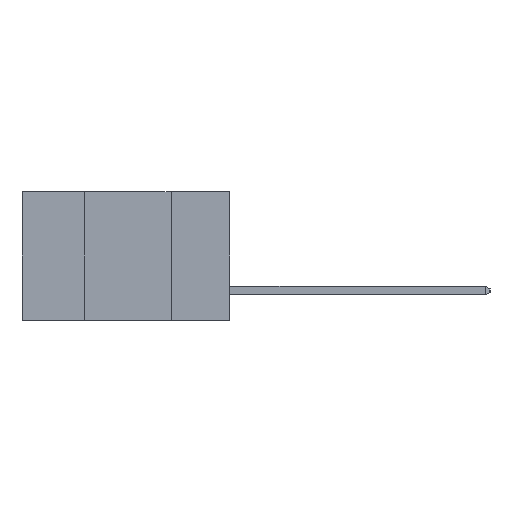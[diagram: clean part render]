
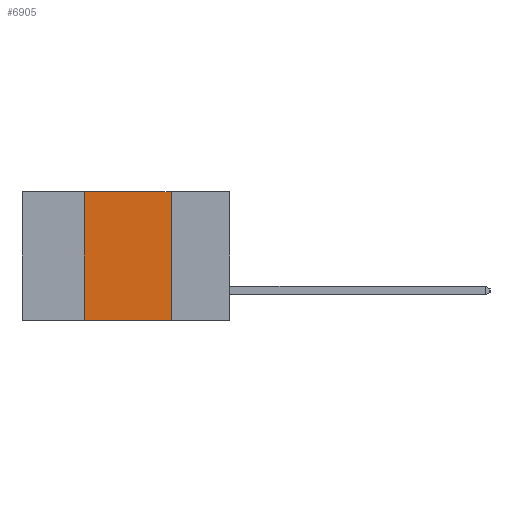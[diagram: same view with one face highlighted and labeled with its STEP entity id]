
A CAD part, left-side view. The second image highlights one B-rep face of the part: STEP entity #6905.
In plain terms, the highlighted planar face has unit normal (-1, 0, 0).
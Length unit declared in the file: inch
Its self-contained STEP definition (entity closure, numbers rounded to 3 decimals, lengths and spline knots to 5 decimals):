
#9 = DIRECTION ( 'NONE',  ( 0., 0., 1. ) ) ;
#81 = DIRECTION ( 'NONE',  ( 0., -1., 0. ) ) ;
#99 = VERTEX_POINT ( 'NONE', #8966 ) ;
#309 = VERTEX_POINT ( 'NONE', #1239 ) ;
#330 = VECTOR ( 'NONE', #81, 39.37008 ) ;
#433 = DIRECTION ( 'NONE',  ( 1., 0., 0. ) ) ;
#480 = DIRECTION ( 'NONE',  ( 0., 0., -1. ) ) ;
#745 = PLANE ( 'NONE',  #10791 ) ;
#835 = EDGE_CURVE ( 'NONE', #309, #99, #3803, .T. ) ;
#1147 = ORIENTED_EDGE ( 'NONE', *, *, #835, .F. ) ;
#1239 = CARTESIAN_POINT ( 'NONE',  ( 0., 0.42, -0.37 ) ) ;
#1526 = EDGE_CURVE ( 'NONE', #309, #7974, #8344, .T. ) ;
#1536 = LINE ( 'NONE', #12085, #8878 ) ;
#1991 = DIRECTION ( 'NONE',  ( 0., -1., 0. ) ) ;
#2173 = ORIENTED_EDGE ( 'NONE', *, *, #10576, .F. ) ;
#2711 = EDGE_LOOP ( 'NONE', ( #2173, #8523, #1147, #6389 ) ) ;
#3203 = VECTOR ( 'NONE', #9, 39.37008 ) ;
#3771 = VECTOR ( 'NONE', #1991, 39.37008 ) ;
#3803 = LINE ( 'NONE', #9398, #3203 ) ;
#4894 = DIRECTION ( 'NONE',  ( 0., 0., -1. ) ) ;
#5002 = CARTESIAN_POINT ( 'NONE',  ( 0., 0.6, 0. ) ) ;
#5019 = CARTESIAN_POINT ( 'NONE',  ( 0., 0.6, 0. ) ) ;
#5763 = CARTESIAN_POINT ( 'NONE',  ( 0., 0.17, 0. ) ) ;
#6086 = FACE_OUTER_BOUND ( 'NONE', #2711, .T. ) ;
#6389 = ORIENTED_EDGE ( 'NONE', *, *, #1526, .T. ) ;
#6905 = ADVANCED_FACE ( 'NONE', ( #6086 ), #745, .F. ) ;
#7974 = VERTEX_POINT ( 'NONE', #11896 ) ;
#8045 = VERTEX_POINT ( 'NONE', #5763 ) ;
#8344 = LINE ( 'NONE', #11282, #330 ) ;
#8523 = ORIENTED_EDGE ( 'NONE', *, *, #8755, .F. ) ;
#8755 = EDGE_CURVE ( 'NONE', #99, #8045, #11089, .T. ) ;
#8878 = VECTOR ( 'NONE', #4894, 39.37008 ) ;
#8966 = CARTESIAN_POINT ( 'NONE',  ( 0., 0.42, 0. ) ) ;
#9398 = CARTESIAN_POINT ( 'NONE',  ( 0., 0.42, 0. ) ) ;
#10576 = EDGE_CURVE ( 'NONE', #8045, #7974, #1536, .T. ) ;
#10791 = AXIS2_PLACEMENT_3D ( 'NONE', #5019, #433, #480 ) ;
#11089 = LINE ( 'NONE', #5002, #3771 ) ;
#11282 = CARTESIAN_POINT ( 'NONE',  ( 0., 0.6, -0.37 ) ) ;
#11896 = CARTESIAN_POINT ( 'NONE',  ( 0., 0.17, -0.37 ) ) ;
#12085 = CARTESIAN_POINT ( 'NONE',  ( 0., 0.17, 0. ) ) ;
